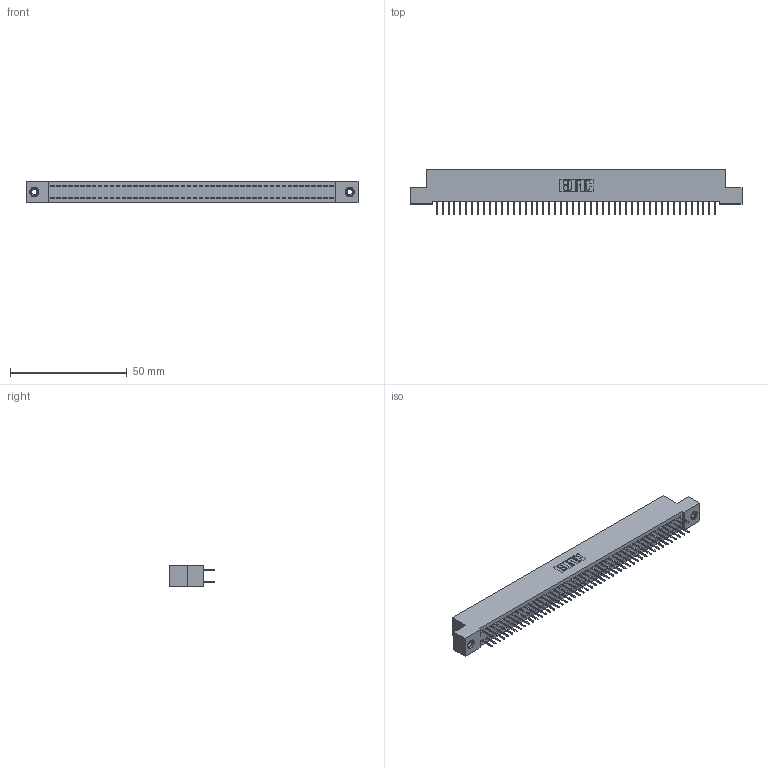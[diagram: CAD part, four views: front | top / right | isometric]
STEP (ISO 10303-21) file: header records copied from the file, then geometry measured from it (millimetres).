
FILE_DESCRIPTION (( 'STEP AP203' ), '1' );
FILE_NAME ('392-096-524-208.STEP', '2019-10-09T19:48:21', ( '' ), ( '' ), 'SwSTEP 2.0', 'SolidWorks 2016', '' );
FILE_SCHEMA (( 'CONFIG_CONTROL_DESIGN' ));
Length unit declared in the file: inch
Products named in the file (4): 342 Part_TI; 345-292-001_345-293-124; 345-250-001_345-250-003-102; 392-096-524-208
Assembly tree (99 placements, depth 2):
  392-096-524-208
    342 Part_TI
    345-292-001_345-293-124  x96
    345-250-001_345-250-003-102  x2
Bounding box: 142.24 x 19.69 x 9.4 mm (x, y, z)
Volume: 12657.7 mm3; surface area: 20383.8 mm2
Topology: 99 solids, 99 shells, 5546 faces, 15699 edges, 10074 vertices
Faces by surface type: plane 4130, cylinder 1400, cone 12, torus 4
Entity records: 31232 total; most frequent: CARTESIAN_POINT 5149, ORIENTED_EDGE 5078, DIRECTION 4421, EDGE_CURVE 2539, LINE 2395, VECTOR 2395, VERTEX_POINT 1684, AXIS2_PLACEMENT_3D 1013
